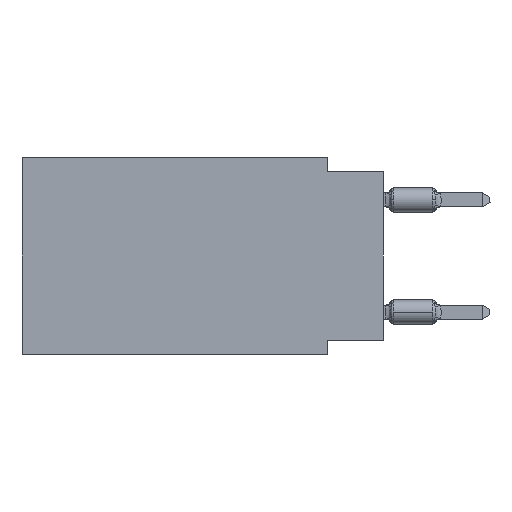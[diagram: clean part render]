
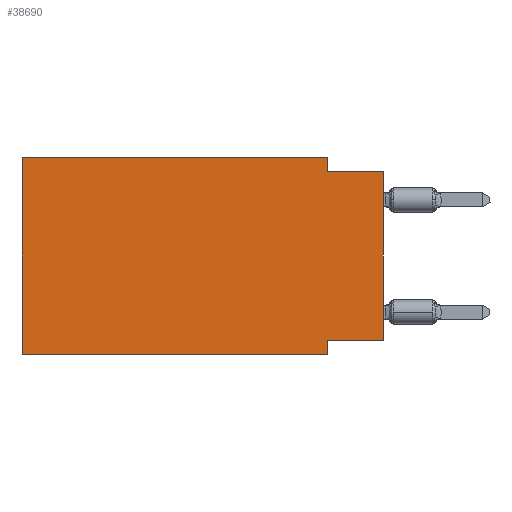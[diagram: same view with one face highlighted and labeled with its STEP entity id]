
A CAD part, left-side view. The second image highlights one B-rep face of the part: STEP entity #38690.
In plain terms, the highlighted planar face has unit normal (-1, 0, 0).
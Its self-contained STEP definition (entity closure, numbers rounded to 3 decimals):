
#901 = CARTESIAN_POINT ( 'NONE',  ( 0., 2.54, -8.89 ) ) ;
#1745 = CARTESIAN_POINT ( 'NONE',  ( 0., 0., -8.255 ) ) ;
#1919 = VECTOR ( 'NONE', #22814, 1000. ) ;
#2130 = CARTESIAN_POINT ( 'NONE',  ( 0., 16.383, 0. ) ) ;
#2208 = EDGE_CURVE ( 'NONE', #35716, #29555, #50912, .T. ) ;
#2925 = EDGE_CURVE ( 'NONE', #59408, #58662, #47814, .T. ) ;
#4729 = CARTESIAN_POINT ( 'NONE',  ( 0., 16.383, 0. ) ) ;
#4962 = EDGE_CURVE ( 'NONE', #45196, #45012, #31093, .T. ) ;
#5802 = CARTESIAN_POINT ( 'NONE',  ( 0., 0., 0. ) ) ;
#6199 = ORIENTED_EDGE ( 'NONE', *, *, #51903, .T. ) ;
#7591 = CARTESIAN_POINT ( 'NONE',  ( 0., 16.383, -8.89 ) ) ;
#9517 = ORIENTED_EDGE ( 'NONE', *, *, #2208, .F. ) ;
#9799 = VECTOR ( 'NONE', #59373, 1000. ) ;
#10132 = FACE_OUTER_BOUND ( 'NONE', #44959, .T. ) ;
#10330 = VECTOR ( 'NONE', #20095, 1000. ) ;
#10681 = CARTESIAN_POINT ( 'NONE',  ( 0., 0., -8.255 ) ) ;
#10881 = ORIENTED_EDGE ( 'NONE', *, *, #11867, .F. ) ;
#11867 = EDGE_CURVE ( 'NONE', #29555, #28693, #50744, .T. ) ;
#12114 = CARTESIAN_POINT ( 'NONE',  ( 0., 0., -0.635 ) ) ;
#12734 = CARTESIAN_POINT ( 'NONE',  ( 0., 2.54, -8.89 ) ) ;
#12761 = ORIENTED_EDGE ( 'NONE', *, *, #2925, .F. ) ;
#14820 = DIRECTION ( 'NONE',  ( 0., 0., 1. ) ) ;
#17930 = CARTESIAN_POINT ( 'NONE',  ( 0., 2.54, -8.255 ) ) ;
#18480 = CARTESIAN_POINT ( 'NONE',  ( 0., 16.383, 0. ) ) ;
#18900 = VECTOR ( 'NONE', #38521, 1000. ) ;
#19713 = AXIS2_PLACEMENT_3D ( 'NONE', #43195, #42907, #42597 ) ;
#20095 = DIRECTION ( 'NONE',  ( 0., 1., 0. ) ) ;
#21130 = LINE ( 'NONE', #7591, #26981 ) ;
#22666 = DIRECTION ( 'NONE',  ( 0., 0., -1. ) ) ;
#22814 = DIRECTION ( 'NONE',  ( 0., -1., 0. ) ) ;
#26981 = VECTOR ( 'NONE', #44265, 1000. ) ;
#27453 = CARTESIAN_POINT ( 'NONE',  ( 0., 16.383, -8.89 ) ) ;
#28209 = CARTESIAN_POINT ( 'NONE',  ( 0., 0., -0.635 ) ) ;
#28464 = EDGE_CURVE ( 'NONE', #58662, #35716, #41036, .T. ) ;
#28693 = VERTEX_POINT ( 'NONE', #12114 ) ;
#29555 = VERTEX_POINT ( 'NONE', #35632 ) ;
#29683 = PLANE ( 'NONE',  #19713 ) ;
#29810 = ORIENTED_EDGE ( 'NONE', *, *, #28464, .F. ) ;
#30765 = ORIENTED_EDGE ( 'NONE', *, *, #55412, .F. ) ;
#31093 = LINE ( 'NONE', #1745, #10330 ) ;
#35632 = CARTESIAN_POINT ( 'NONE',  ( 0., 2.54, -0.635 ) ) ;
#35716 = VERTEX_POINT ( 'NONE', #42732 ) ;
#36498 = CARTESIAN_POINT ( 'NONE',  ( 0., 2.54, 0. ) ) ;
#37878 = VECTOR ( 'NONE', #22666, 1000. ) ;
#38163 = VERTEX_POINT ( 'NONE', #901 ) ;
#38521 = DIRECTION ( 'NONE',  ( 0., 0., 1. ) ) ;
#38690 = ADVANCED_FACE ( 'NONE', ( #10132 ), #29683, .F. ) ;
#40883 = EDGE_CURVE ( 'NONE', #45196, #28693, #47573, .T. ) ;
#41036 = LINE ( 'NONE', #18480, #9799 ) ;
#42597 = DIRECTION ( 'NONE',  ( 0., 0., -1. ) ) ;
#42732 = CARTESIAN_POINT ( 'NONE',  ( 0., 2.54, 0. ) ) ;
#42907 = DIRECTION ( 'NONE',  ( 1., 0., 0. ) ) ;
#43195 = CARTESIAN_POINT ( 'NONE',  ( 0., 16.383, 0. ) ) ;
#43908 = VECTOR ( 'NONE', #14820, 1000. ) ;
#44123 = ORIENTED_EDGE ( 'NONE', *, *, #4962, .F. ) ;
#44265 = DIRECTION ( 'NONE',  ( 0., -1., 0. ) ) ;
#44959 = EDGE_LOOP ( 'NONE', ( #46082, #10881, #9517, #29810, #12761, #6199, #30765, #44123 ) ) ;
#45012 = VERTEX_POINT ( 'NONE', #17930 ) ;
#45196 = VERTEX_POINT ( 'NONE', #10681 ) ;
#46082 = ORIENTED_EDGE ( 'NONE', *, *, #40883, .T. ) ;
#47573 = LINE ( 'NONE', #5802, #43908 ) ;
#47814 = LINE ( 'NONE', #2130, #18900 ) ;
#50744 = LINE ( 'NONE', #28209, #1919 ) ;
#50912 = LINE ( 'NONE', #36498, #51435 ) ;
#51435 = VECTOR ( 'NONE', #55129, 1000. ) ;
#51903 = EDGE_CURVE ( 'NONE', #59408, #38163, #21130, .T. ) ;
#54815 = LINE ( 'NONE', #12734, #37878 ) ;
#55129 = DIRECTION ( 'NONE',  ( 0., 0., -1. ) ) ;
#55412 = EDGE_CURVE ( 'NONE', #45012, #38163, #54815, .T. ) ;
#58662 = VERTEX_POINT ( 'NONE', #4729 ) ;
#59373 = DIRECTION ( 'NONE',  ( 0., -1., 0. ) ) ;
#59408 = VERTEX_POINT ( 'NONE', #27453 ) ;
